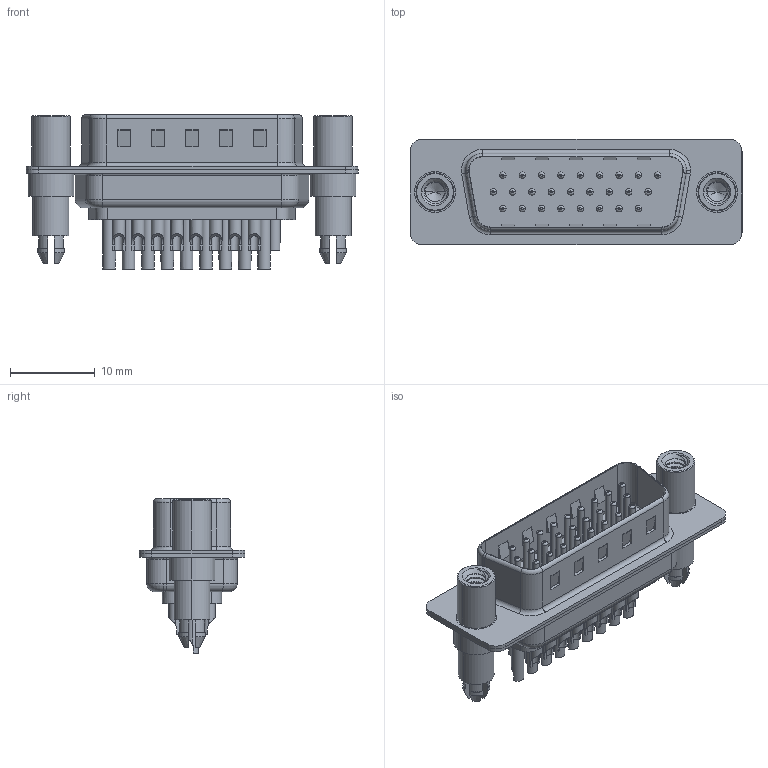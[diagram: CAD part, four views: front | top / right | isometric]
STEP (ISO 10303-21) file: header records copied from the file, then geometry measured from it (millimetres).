
FILE_DESCRIPTION (( 'STEP AP203' ), '1' );
FILE_NAME ('637-M26-632-BN6.STEP', '2018-11-20T00:20:24', ( '' ), ( '' ), 'SwSTEP 2.0', 'SolidWorks 2016', '' );
FILE_SCHEMA (( 'CONFIG_CONTROL_DESIGN' ));
Length unit declared in the file: millimetre
Products named in the file (8): 637M Shell Rear_26 Contacts; 637M Contact Row 1_32; 637M Contact Row 2_32; 637M Contact Row 3_32; 637M 4-40 Threaded Standoff and Boardlock; 637-M26-632-BN6; 637M Housing_26 Contacts; 637M Shell Front_26 Contacts
Assembly tree (31 placements, depth 2):
  637-M26-632-BN6
    637M Housing_26 Contacts
    637M Shell Front_26 Contacts
    637M Shell Rear_26 Contacts
    637M Contact Row 1_32  x9
    637M Contact Row 2_32  x9
    637M Contact Row 3_32  x8
    637M 4-40 Threaded Standoff and Boardlock  x2
Bounding box: 39.2 x 12.5 x 18.25 mm (x, y, z)
Volume: 2332.5 mm3; surface area: 6557.7 mm2
Topology: 31 solids, 31 shells, 1386 faces, 3253 edges, 2002 vertices
Faces by surface type: cylinder 585, plane 411, torus 310, cone 74, bspline 6
Entity records: 21668 total; most frequent: CARTESIAN_POINT 4533, DIRECTION 3513, ORIENTED_EDGE 3080, EDGE_CURVE 1540, AXIS2_PLACEMENT_3D 1396, VERTEX_POINT 984, EDGE_LOOP 802, CIRCLE 721
